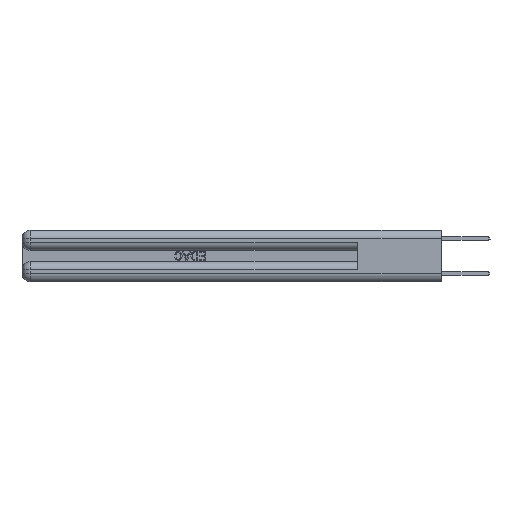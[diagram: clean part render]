
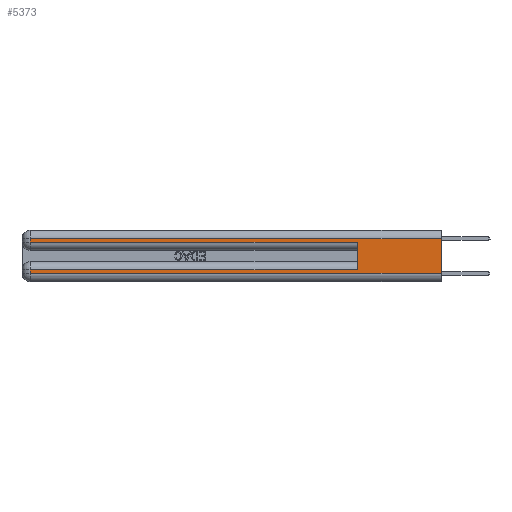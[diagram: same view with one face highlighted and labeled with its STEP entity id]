
A CAD part, left-side view. The second image highlights one B-rep face of the part: STEP entity #5373.
In plain terms, the highlighted planar face has unit normal (-1, 0, 0).
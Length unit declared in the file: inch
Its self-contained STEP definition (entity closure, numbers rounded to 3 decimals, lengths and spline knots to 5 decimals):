
#1040 = CARTESIAN_POINT ( 'NONE',  ( 0., 2.94, 0.085 ) ) ;
#1348 = EDGE_CURVE ( 'NONE', #19900, #19343, #24965, .T. ) ;
#2017 = LINE ( 'NONE', #22197, #8309 ) ;
#2381 = CARTESIAN_POINT ( 'NONE',  ( 0., 0., 0.31 ) ) ;
#3538 = VERTEX_POINT ( 'NONE', #14696 ) ;
#3907 = DIRECTION ( 'NONE',  ( 0., 0., -1. ) ) ;
#3998 = EDGE_LOOP ( 'NONE', ( #9955, #4223, #18106, #25994, #7369, #8016, #11971, #28730 ) ) ;
#4005 = VECTOR ( 'NONE', #28543, 39.37008 ) ;
#4091 = PLANE ( 'NONE',  #23711 ) ;
#4223 = ORIENTED_EDGE ( 'NONE', *, *, #22266, .T. ) ;
#4326 = VECTOR ( 'NONE', #7810, 39.37008 ) ;
#5216 = VERTEX_POINT ( 'NONE', #13077 ) ;
#5308 = LINE ( 'NONE', #24903, #19292 ) ;
#5373 = ADVANCED_FACE ( 'NONE', ( #25118 ), #4091, .F. ) ;
#5600 = DIRECTION ( 'NONE',  ( 0., -1., 0. ) ) ;
#6868 = LINE ( 'NONE', #24496, #22380 ) ;
#7039 = DIRECTION ( 'NONE',  ( 0., 1., 0. ) ) ;
#7369 = ORIENTED_EDGE ( 'NONE', *, *, #17871, .F. ) ;
#7810 = DIRECTION ( 'NONE',  ( 0., 0., -1. ) ) ;
#8016 = ORIENTED_EDGE ( 'NONE', *, *, #29147, .T. ) ;
#8071 = VERTEX_POINT ( 'NONE', #13029 ) ;
#8309 = VECTOR ( 'NONE', #5600, 39.37008 ) ;
#9174 = LINE ( 'NONE', #14793, #4005 ) ;
#9955 = ORIENTED_EDGE ( 'NONE', *, *, #1348, .F. ) ;
#11120 = CARTESIAN_POINT ( 'NONE',  ( 0., 0., 0.37 ) ) ;
#11971 = ORIENTED_EDGE ( 'NONE', *, *, #16335, .T. ) ;
#12945 = LINE ( 'NONE', #25647, #26929 ) ;
#13029 = CARTESIAN_POINT ( 'NONE',  ( 0., 2.94, 0.06 ) ) ;
#13077 = CARTESIAN_POINT ( 'NONE',  ( 0., 0.6, 0.085 ) ) ;
#13392 = DIRECTION ( 'NONE',  ( 1., 0., 0. ) ) ;
#14696 = CARTESIAN_POINT ( 'NONE',  ( 0., 2.94, 0.31 ) ) ;
#14793 = CARTESIAN_POINT ( 'NONE',  ( 0., 2.94, 0.37 ) ) ;
#14879 = CARTESIAN_POINT ( 'NONE',  ( 0., 0., 0.37 ) ) ;
#15021 = DIRECTION ( 'NONE',  ( 0., 0., 1. ) ) ;
#15238 = VERTEX_POINT ( 'NONE', #20030 ) ;
#16335 = EDGE_CURVE ( 'NONE', #18489, #8071, #9174, .T. ) ;
#17562 = VECTOR ( 'NONE', #7039, 39.37008 ) ;
#17871 = EDGE_CURVE ( 'NONE', #5216, #23946, #6868, .T. ) ;
#17917 = CARTESIAN_POINT ( 'NONE',  ( 0., 0., 0.31 ) ) ;
#18106 = ORIENTED_EDGE ( 'NONE', *, *, #23469, .T. ) ;
#18143 = DIRECTION ( 'NONE',  ( 0., 1., 0. ) ) ;
#18489 = VERTEX_POINT ( 'NONE', #1040 ) ;
#19292 = VECTOR ( 'NONE', #3907, 39.37008 ) ;
#19343 = VERTEX_POINT ( 'NONE', #23879 ) ;
#19900 = VERTEX_POINT ( 'NONE', #17917 ) ;
#19948 = CARTESIAN_POINT ( 'NONE',  ( 0., 0.6, 0.285 ) ) ;
#20030 = CARTESIAN_POINT ( 'NONE',  ( 0., 2.94, 0.285 ) ) ;
#20297 = CARTESIAN_POINT ( 'NONE',  ( 0., 0., 0.085 ) ) ;
#22197 = CARTESIAN_POINT ( 'NONE',  ( 0., 0., 0.06 ) ) ;
#22266 = EDGE_CURVE ( 'NONE', #19900, #3538, #24453, .T. ) ;
#22380 = VECTOR ( 'NONE', #15021, 39.37008 ) ;
#22579 = EDGE_CURVE ( 'NONE', #8071, #19343, #2017, .T. ) ;
#23469 = EDGE_CURVE ( 'NONE', #3538, #15238, #5308, .T. ) ;
#23711 = AXIS2_PLACEMENT_3D ( 'NONE', #11120, #13392, #25090 ) ;
#23724 = VECTOR ( 'NONE', #18143, 39.37008 ) ;
#23879 = CARTESIAN_POINT ( 'NONE',  ( 0., 0., 0.06 ) ) ;
#23946 = VERTEX_POINT ( 'NONE', #19948 ) ;
#24453 = LINE ( 'NONE', #2381, #17562 ) ;
#24496 = CARTESIAN_POINT ( 'NONE',  ( 0., 0.6, 0.145 ) ) ;
#24903 = CARTESIAN_POINT ( 'NONE',  ( 0., 2.94, 0.37 ) ) ;
#24965 = LINE ( 'NONE', #14879, #4326 ) ;
#25090 = DIRECTION ( 'NONE',  ( 0., 0., -1. ) ) ;
#25118 = FACE_OUTER_BOUND ( 'NONE', #3998, .T. ) ;
#25415 = EDGE_CURVE ( 'NONE', #15238, #23946, #12945, .T. ) ;
#25647 = CARTESIAN_POINT ( 'NONE',  ( 0., 0., 0.285 ) ) ;
#25994 = ORIENTED_EDGE ( 'NONE', *, *, #25415, .T. ) ;
#26929 = VECTOR ( 'NONE', #28250, 39.37008 ) ;
#28250 = DIRECTION ( 'NONE',  ( 0., -1., 0. ) ) ;
#28543 = DIRECTION ( 'NONE',  ( 0., 0., -1. ) ) ;
#28730 = ORIENTED_EDGE ( 'NONE', *, *, #22579, .T. ) ;
#29147 = EDGE_CURVE ( 'NONE', #5216, #18489, #30040, .T. ) ;
#30040 = LINE ( 'NONE', #20297, #23724 ) ;
